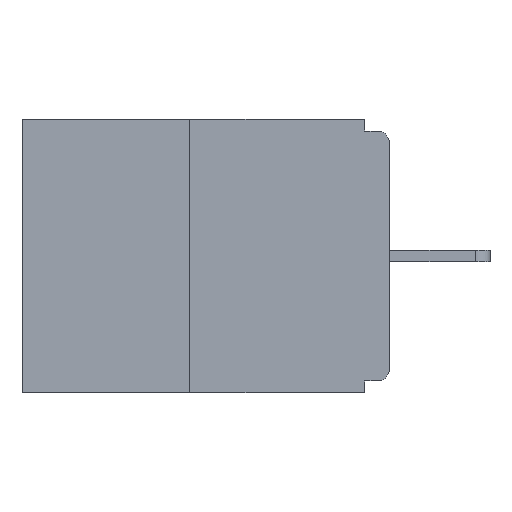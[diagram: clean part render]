
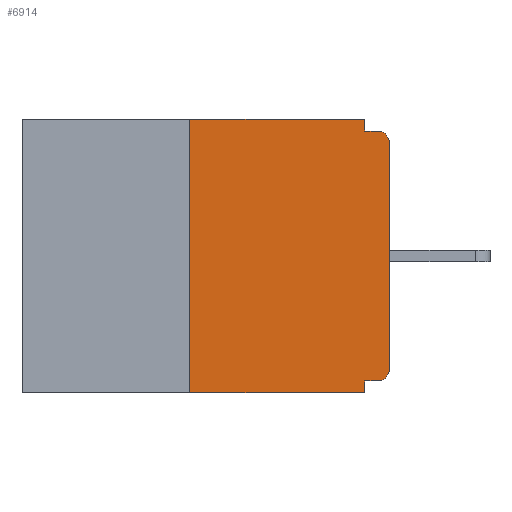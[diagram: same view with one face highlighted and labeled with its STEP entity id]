
A CAD part, left-side view. The second image highlights one B-rep face of the part: STEP entity #6914.
In plain terms, the highlighted planar face has unit normal (-1, 0, 0).
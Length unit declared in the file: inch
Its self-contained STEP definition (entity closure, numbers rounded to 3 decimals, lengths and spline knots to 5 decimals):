
#397 = CARTESIAN_POINT ( 'NONE',  ( 0., 0., -0.015 ) ) ;
#892 = DIRECTION ( 'NONE',  ( 0., 0., 1. ) ) ;
#1244 = VERTEX_POINT ( 'NONE', #11782 ) ;
#1530 = AXIS2_PLACEMENT_3D ( 'NONE', #14111, #5540, #15503 ) ;
#1914 = DIRECTION ( 'NONE',  ( 0., -1., 0. ) ) ;
#2123 = ORIENTED_EDGE ( 'NONE', *, *, #3389, .T. ) ;
#2362 = CARTESIAN_POINT ( 'NONE',  ( 0., 0.031, -0.343 ) ) ;
#2382 = DIRECTION ( 'NONE',  ( 0., 0., -1. ) ) ;
#2444 = VECTOR ( 'NONE', #892, 39.37008 ) ;
#2467 = LINE ( 'NONE', #13662, #14480 ) ;
#2532 = VECTOR ( 'NONE', #13608, 39.37008 ) ;
#2574 = EDGE_LOOP ( 'NONE', ( #6055, #8109, #9727, #7716, #5876, #2123, #7969, #6822, #15483, #13976 ) ) ;
#2938 = AXIS2_PLACEMENT_3D ( 'NONE', #6239, #16172, #7734 ) ;
#3014 = CARTESIAN_POINT ( 'NONE',  ( 0., 0.031, -0.015 ) ) ;
#3106 = VERTEX_POINT ( 'NONE', #8380 ) ;
#3389 = EDGE_CURVE ( 'NONE', #13526, #1244, #14374, .T. ) ;
#3415 = VECTOR ( 'NONE', #9787, 39.37008 ) ;
#3476 = CARTESIAN_POINT ( 'NONE',  ( 0., 0., -0.328 ) ) ;
#3946 = LINE ( 'NONE', #397, #11249 ) ;
#4642 = LINE ( 'NONE', #15642, #12353 ) ;
#4719 = CARTESIAN_POINT ( 'NONE',  ( 0., 0.015, -0.328 ) ) ;
#4833 = FACE_OUTER_BOUND ( 'NONE', #2574, .T. ) ;
#5046 = DIRECTION ( 'NONE',  ( 0., 0., 1. ) ) ;
#5079 = CARTESIAN_POINT ( 'NONE',  ( 0., 0.015, -0.313 ) ) ;
#5171 = CARTESIAN_POINT ( 'NONE',  ( 0., 0.25, 0. ) ) ;
#5540 = DIRECTION ( 'NONE',  ( -1., 0., 0. ) ) ;
#5732 = EDGE_CURVE ( 'NONE', #13526, #11526, #13664, .T. ) ;
#5876 = ORIENTED_EDGE ( 'NONE', *, *, #5732, .F. ) ;
#6055 = ORIENTED_EDGE ( 'NONE', *, *, #13991, .F. ) ;
#6204 = VERTEX_POINT ( 'NONE', #3014 ) ;
#6239 = CARTESIAN_POINT ( 'NONE',  ( 0., 0.46, 0. ) ) ;
#6425 = CIRCLE ( 'NONE', #1530, 0.015 ) ;
#6652 = DIRECTION ( 'NONE',  ( -1., 0., 0. ) ) ;
#6694 = DIRECTION ( 'NONE',  ( 0., 0., -1. ) ) ;
#6822 = ORIENTED_EDGE ( 'NONE', *, *, #12199, .T. ) ;
#6914 = ADVANCED_FACE ( 'NONE', ( #4833 ), #10528, .F. ) ;
#7028 = CARTESIAN_POINT ( 'NONE',  ( 0., 0., -0.03 ) ) ;
#7393 = LINE ( 'NONE', #8351, #3415 ) ;
#7665 = LINE ( 'NONE', #11620, #18394 ) ;
#7716 = ORIENTED_EDGE ( 'NONE', *, *, #10822, .F. ) ;
#7734 = DIRECTION ( 'NONE',  ( 0., 0., -1. ) ) ;
#7969 = ORIENTED_EDGE ( 'NONE', *, *, #15918, .T. ) ;
#8109 = ORIENTED_EDGE ( 'NONE', *, *, #15516, .F. ) ;
#8260 = VERTEX_POINT ( 'NONE', #16971 ) ;
#8351 = CARTESIAN_POINT ( 'NONE',  ( 0., 0.46, -0.343 ) ) ;
#8380 = CARTESIAN_POINT ( 'NONE',  ( 0., 0.031, -0.343 ) ) ;
#8569 = CARTESIAN_POINT ( 'NONE',  ( 0., 0.015, -0.015 ) ) ;
#8944 = VERTEX_POINT ( 'NONE', #8569 ) ;
#9244 = EDGE_CURVE ( 'NONE', #6204, #8944, #3946, .T. ) ;
#9426 = EDGE_CURVE ( 'NONE', #15727, #6204, #4642, .T. ) ;
#9727 = ORIENTED_EDGE ( 'NONE', *, *, #15058, .T. ) ;
#9787 = DIRECTION ( 'NONE',  ( 0., -1., 0. ) ) ;
#10262 = LINE ( 'NONE', #18101, #2444 ) ;
#10528 = PLANE ( 'NONE',  #2938 ) ;
#10750 = LINE ( 'NONE', #2362, #17722 ) ;
#10822 = EDGE_CURVE ( 'NONE', #11526, #3106, #10750, .T. ) ;
#11249 = VECTOR ( 'NONE', #1914, 39.37008 ) ;
#11402 = VERTEX_POINT ( 'NONE', #5171 ) ;
#11526 = VERTEX_POINT ( 'NONE', #18215 ) ;
#11620 = CARTESIAN_POINT ( 'NONE',  ( 0., 0.46, 0. ) ) ;
#11782 = CARTESIAN_POINT ( 'NONE',  ( 0., 0., -0.313 ) ) ;
#12199 = EDGE_CURVE ( 'NONE', #18306, #8944, #6425, .T. ) ;
#12353 = VECTOR ( 'NONE', #2382, 39.37008 ) ;
#12680 = CARTESIAN_POINT ( 'NONE',  ( 0., 0.031, 0. ) ) ;
#13526 = VERTEX_POINT ( 'NONE', #4719 ) ;
#13608 = DIRECTION ( 'NONE',  ( 0., 1., 0. ) ) ;
#13662 = CARTESIAN_POINT ( 'NONE',  ( 0., 0.25, 0. ) ) ;
#13664 = LINE ( 'NONE', #3476, #2532 ) ;
#13976 = ORIENTED_EDGE ( 'NONE', *, *, #9426, .F. ) ;
#13991 = EDGE_CURVE ( 'NONE', #11402, #15727, #7665, .T. ) ;
#14111 = CARTESIAN_POINT ( 'NONE',  ( 0., 0.015, -0.03 ) ) ;
#14374 = CIRCLE ( 'NONE', #15316, 0.015 ) ;
#14480 = VECTOR ( 'NONE', #5046, 39.37008 ) ;
#15058 = EDGE_CURVE ( 'NONE', #8260, #3106, #7393, .T. ) ;
#15316 = AXIS2_PLACEMENT_3D ( 'NONE', #5079, #6652, #6694 ) ;
#15483 = ORIENTED_EDGE ( 'NONE', *, *, #9244, .F. ) ;
#15503 = DIRECTION ( 'NONE',  ( 0., 0., -1. ) ) ;
#15516 = EDGE_CURVE ( 'NONE', #8260, #11402, #2467, .T. ) ;
#15642 = CARTESIAN_POINT ( 'NONE',  ( 0., 0.031, 0. ) ) ;
#15727 = VERTEX_POINT ( 'NONE', #12680 ) ;
#15840 = DIRECTION ( 'NONE',  ( 0., -1., 0. ) ) ;
#15918 = EDGE_CURVE ( 'NONE', #1244, #18306, #10262, .T. ) ;
#16172 = DIRECTION ( 'NONE',  ( 1., 0., 0. ) ) ;
#16739 = DIRECTION ( 'NONE',  ( 0., 0., -1. ) ) ;
#16971 = CARTESIAN_POINT ( 'NONE',  ( 0., 0.25, -0.343 ) ) ;
#17722 = VECTOR ( 'NONE', #16739, 39.37008 ) ;
#18101 = CARTESIAN_POINT ( 'NONE',  ( 0., 0., 0. ) ) ;
#18215 = CARTESIAN_POINT ( 'NONE',  ( 0., 0.031, -0.328 ) ) ;
#18306 = VERTEX_POINT ( 'NONE', #7028 ) ;
#18394 = VECTOR ( 'NONE', #15840, 39.37008 ) ;
